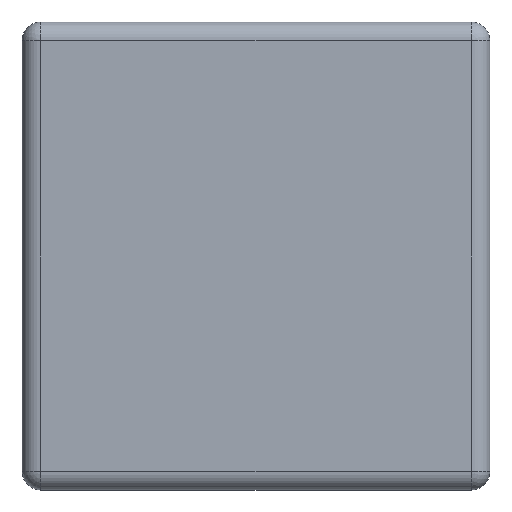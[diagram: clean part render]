
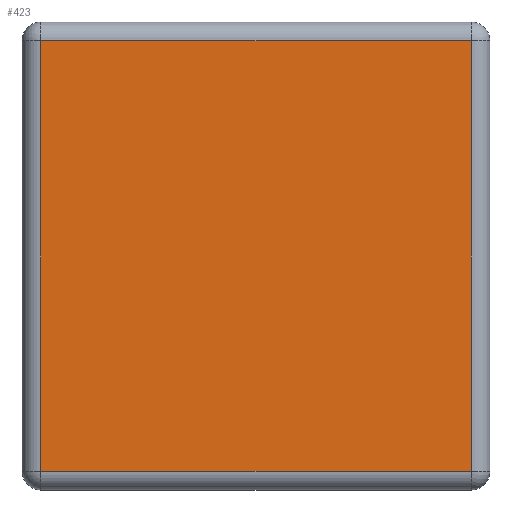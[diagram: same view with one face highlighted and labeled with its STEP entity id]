
A CAD part, front view. The second image highlights one B-rep face of the part: STEP entity #423.
In plain terms, the highlighted planar face has unit normal (0, -1, 0).
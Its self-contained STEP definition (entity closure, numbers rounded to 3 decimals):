
#26=PLANE('',#499);
#32=LINE('',#779,#57);
#34=LINE('',#789,#59);
#36=LINE('',#792,#61);
#46=LINE('',#807,#71);
#57=VECTOR('',#589,10.);
#59=VECTOR('',#601,10.);
#61=VECTOR('',#605,10.);
#71=VECTOR('',#625,10.);
#122=FACE_OUTER_BOUND('',#153,.T.);
#153=EDGE_LOOP('',(#375,#376,#377,#378));
#204=VERTEX_POINT('',#744);
#212=VERTEX_POINT('',#761);
#218=VERTEX_POINT('',#775);
#221=VERTEX_POINT('',#785);
#253=EDGE_CURVE('',#204,#218,#32,.T.);
#258=EDGE_CURVE('',#218,#221,#34,.T.);
#260=EDGE_CURVE('',#221,#212,#36,.T.);
#270=EDGE_CURVE('',#212,#204,#46,.T.);
#375=ORIENTED_EDGE('',*,*,#253,.F.);
#376=ORIENTED_EDGE('',*,*,#270,.F.);
#377=ORIENTED_EDGE('',*,*,#260,.F.);
#378=ORIENTED_EDGE('',*,*,#258,.F.);
#423=ADVANCED_FACE('',(#122),#26,.F.);
#499=AXIS2_PLACEMENT_3D('',#822,#645,#646);
#589=DIRECTION('',(1.,0.,0.));
#601=DIRECTION('',(0.,0.,-1.));
#605=DIRECTION('',(-1.,0.,0.));
#625=DIRECTION('',(0.,0.,1.));
#645=DIRECTION('center_axis',(0.,1.,0.));
#646=DIRECTION('ref_axis',(1.,0.,0.));
#744=CARTESIAN_POINT('',(178.18,112.159,13.632));
#761=CARTESIAN_POINT('',(178.18,112.159,-32.368));
#775=CARTESIAN_POINT('',(224.18,112.159,13.632));
#779=CARTESIAN_POINT('',(188.68,112.159,13.632));
#785=CARTESIAN_POINT('',(224.18,112.159,-32.368));
#789=CARTESIAN_POINT('',(224.18,112.159,3.132));
#792=CARTESIAN_POINT('',(213.68,112.159,-32.368));
#807=CARTESIAN_POINT('',(178.18,112.159,-21.868));
#822=CARTESIAN_POINT('Origin',(201.18,112.159,-9.368));
